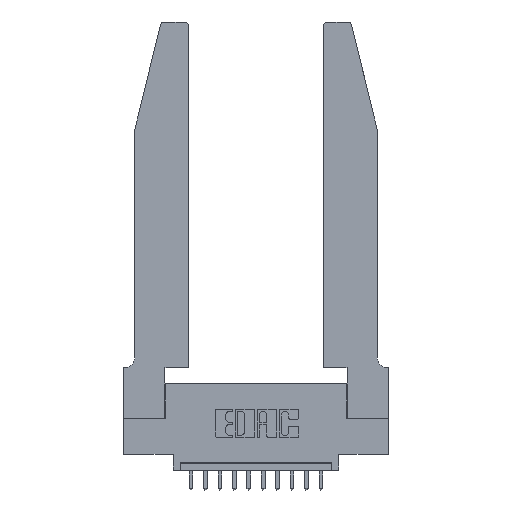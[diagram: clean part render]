
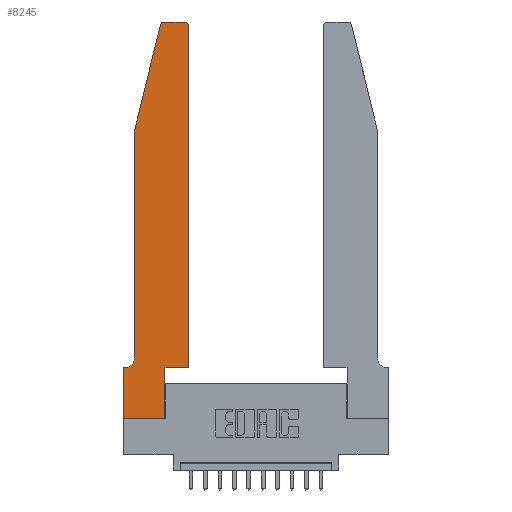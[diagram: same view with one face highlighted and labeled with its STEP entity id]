
A CAD part, top view. The second image highlights one B-rep face of the part: STEP entity #8245.
In plain terms, the highlighted planar face has unit normal (0, 0, 1).
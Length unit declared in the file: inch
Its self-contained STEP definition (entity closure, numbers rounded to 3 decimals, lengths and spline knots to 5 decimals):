
#214 = ORIENTED_EDGE ( 'NONE', *, *, #12427, .T. ) ;
#364 = CARTESIAN_POINT ( 'NONE',  ( 0.0755, 2., 0.37 ) ) ;
#446 = DIRECTION ( 'NONE',  ( -1., 0., 0. ) ) ;
#519 = EDGE_CURVE ( 'NONE', #14532, #1285, #1143, .T. ) ;
#826 = VERTEX_POINT ( 'NONE', #7293 ) ;
#1064 = VECTOR ( 'NONE', #11147, 39.37008 ) ;
#1143 = LINE ( 'NONE', #16599, #11051 ) ;
#1285 = VERTEX_POINT ( 'NONE', #364 ) ;
#1430 = VERTEX_POINT ( 'NONE', #10833 ) ;
#1676 = ORIENTED_EDGE ( 'NONE', *, *, #519, .T. ) ;
#1747 = DIRECTION ( 'NONE',  ( 1., 0., 0. ) ) ;
#1871 = DIRECTION ( 'NONE',  ( 0., 0., -1. ) ) ;
#1930 = VERTEX_POINT ( 'NONE', #14676 ) ;
#2020 = EDGE_CURVE ( 'NONE', #9613, #1430, #5554, .T. ) ;
#2262 = EDGE_CURVE ( 'NONE', #9826, #11814, #2734, .T. ) ;
#2315 = VECTOR ( 'NONE', #14000, 39.37008 ) ;
#2559 = DIRECTION ( 'NONE',  ( -0.239, -0.971, 0. ) ) ;
#2623 = CARTESIAN_POINT ( 'NONE',  ( 0.4505, 0.35, 0.37 ) ) ;
#2734 = LINE ( 'NONE', #5154, #2315 ) ;
#2771 = EDGE_CURVE ( 'NONE', #14630, #3129, #10166, .T. ) ;
#3014 = EDGE_CURVE ( 'NONE', #826, #9613, #12371, .T. ) ;
#3129 = VERTEX_POINT ( 'NONE', #7586 ) ;
#3206 = ORIENTED_EDGE ( 'NONE', *, *, #6426, .T. ) ;
#3350 = CARTESIAN_POINT ( 'NONE',  ( 0., 0., 0.37 ) ) ;
#3402 = LINE ( 'NONE', #9365, #4191 ) ;
#3431 = CARTESIAN_POINT ( 'NONE',  ( 0.25487, 2.72718, 0.37 ) ) ;
#3450 = EDGE_LOOP ( 'NONE', ( #13868, #10071, #1676, #14899, #9707, #16537, #13257, #11878, #3206, #13038, #214, #4531 ) ) ;
#3834 = VECTOR ( 'NONE', #12925, 39.37008 ) ;
#3857 = CARTESIAN_POINT ( 'NONE',  ( 0., 0.35, 0.37 ) ) ;
#3971 = CARTESIAN_POINT ( 'NONE',  ( 0.4205, 2.72, 0.37 ) ) ;
#4080 = DIRECTION ( 'NONE',  ( 0., 0., 1. ) ) ;
#4191 = VECTOR ( 'NONE', #446, 39.37008 ) ;
#4404 = EDGE_CURVE ( 'NONE', #1285, #1930, #16577, .T. ) ;
#4475 = DIRECTION ( 'NONE',  ( -1., 0., 0. ) ) ;
#4479 = CARTESIAN_POINT ( 'NONE',  ( 0., 0., 0.37 ) ) ;
#4531 = ORIENTED_EDGE ( 'NONE', *, *, #2771, .T. ) ;
#4622 = DIRECTION ( 'NONE',  ( 0., 1., 0. ) ) ;
#4669 = LINE ( 'NONE', #2623, #3834 ) ;
#5014 = DIRECTION ( 'NONE',  ( 0., 0., 1. ) ) ;
#5154 = CARTESIAN_POINT ( 'NONE',  ( 0.4505, 0.35, 0.37 ) ) ;
#5554 = LINE ( 'NONE', #3350, #15008 ) ;
#5591 = CARTESIAN_POINT ( 'NONE',  ( 0.4505, 0.35, 0.37 ) ) ;
#5852 = DIRECTION ( 'NONE',  ( 1., 0., 0. ) ) ;
#6157 = CARTESIAN_POINT ( 'NONE',  ( 0.2865, 0.35, 0.37 ) ) ;
#6426 = EDGE_CURVE ( 'NONE', #1430, #9826, #13929, .T. ) ;
#6497 = AXIS2_PLACEMENT_3D ( 'NONE', #14771, #1871, #4475 ) ;
#7072 = EDGE_CURVE ( 'NONE', #3129, #7613, #3402, .T. ) ;
#7178 = CARTESIAN_POINT ( 'NONE',  ( 0.2865, 0.35, 0.37 ) ) ;
#7293 = CARTESIAN_POINT ( 'NONE',  ( 0., 0.35, 0.37 ) ) ;
#7442 = DIRECTION ( 'NONE',  ( -1., 0., 0. ) ) ;
#7586 = CARTESIAN_POINT ( 'NONE',  ( 0.4205, 2.75, 0.37 ) ) ;
#7613 = VERTEX_POINT ( 'NONE', #16133 ) ;
#8162 = CIRCLE ( 'NONE', #6497, 0.07 ) ;
#8190 = CARTESIAN_POINT ( 'NONE',  ( 0.284, 2.72, 0.37 ) ) ;
#8245 = ADVANCED_FACE ( 'NONE', ( #15655 ), #9014, .T. ) ;
#8492 = VECTOR ( 'NONE', #12927, 39.37008 ) ;
#9014 = PLANE ( 'NONE',  #12389 ) ;
#9365 = CARTESIAN_POINT ( 'NONE',  ( 0.2605, 2.75, 0.37 ) ) ;
#9613 = VERTEX_POINT ( 'NONE', #14556 ) ;
#9707 = ORIENTED_EDGE ( 'NONE', *, *, #15686, .T. ) ;
#9826 = VERTEX_POINT ( 'NONE', #6157 ) ;
#9971 = CARTESIAN_POINT ( 'NONE',  ( 0.0755, 0.35, 0.37 ) ) ;
#10071 = ORIENTED_EDGE ( 'NONE', *, *, #15635, .T. ) ;
#10166 = CIRCLE ( 'NONE', #13939, 0.03 ) ;
#10833 = CARTESIAN_POINT ( 'NONE',  ( 0.2865, 0., 0.37 ) ) ;
#11051 = VECTOR ( 'NONE', #2559, 39.37008 ) ;
#11102 = VECTOR ( 'NONE', #4622, 39.37008 ) ;
#11147 = DIRECTION ( 'NONE',  ( 0., -1., 0. ) ) ;
#11606 = CIRCLE ( 'NONE', #14357, 0.03 ) ;
#11757 = CARTESIAN_POINT ( 'NONE',  ( 0.0755, 2., 0.37 ) ) ;
#11814 = VERTEX_POINT ( 'NONE', #5591 ) ;
#11878 = ORIENTED_EDGE ( 'NONE', *, *, #2020, .T. ) ;
#12342 = CARTESIAN_POINT ( 'NONE',  ( 0.0055, 0.35, 0.37 ) ) ;
#12371 = LINE ( 'NONE', #4479, #1064 ) ;
#12389 = AXIS2_PLACEMENT_3D ( 'NONE', #3857, #5014, #16685 ) ;
#12427 = EDGE_CURVE ( 'NONE', #11814, #14630, #4669, .T. ) ;
#12925 = DIRECTION ( 'NONE',  ( 0., 1., 0. ) ) ;
#12927 = DIRECTION ( 'NONE',  ( 0., -1., 0. ) ) ;
#13038 = ORIENTED_EDGE ( 'NONE', *, *, #2262, .T. ) ;
#13257 = ORIENTED_EDGE ( 'NONE', *, *, #3014, .T. ) ;
#13438 = DIRECTION ( 'NONE',  ( 0., 0., 1. ) ) ;
#13712 = CARTESIAN_POINT ( 'NONE',  ( 0.4505, 2.72, 0.37 ) ) ;
#13868 = ORIENTED_EDGE ( 'NONE', *, *, #7072, .T. ) ;
#13929 = LINE ( 'NONE', #7178, #11102 ) ;
#13939 = AXIS2_PLACEMENT_3D ( 'NONE', #3971, #4080, #14350 ) ;
#14000 = DIRECTION ( 'NONE',  ( 1., 0., 0. ) ) ;
#14048 = LINE ( 'NONE', #9971, #15449 ) ;
#14350 = DIRECTION ( 'NONE',  ( 1., 0., 0. ) ) ;
#14357 = AXIS2_PLACEMENT_3D ( 'NONE', #8190, #13438, #1747 ) ;
#14532 = VERTEX_POINT ( 'NONE', #3431 ) ;
#14556 = CARTESIAN_POINT ( 'NONE',  ( 0., 0., 0.37 ) ) ;
#14630 = VERTEX_POINT ( 'NONE', #13712 ) ;
#14676 = CARTESIAN_POINT ( 'NONE',  ( 0.0755, 0.42, 0.37 ) ) ;
#14771 = CARTESIAN_POINT ( 'NONE',  ( 0.0055, 0.42, 0.37 ) ) ;
#14792 = EDGE_CURVE ( 'NONE', #16671, #826, #14048, .T. ) ;
#14899 = ORIENTED_EDGE ( 'NONE', *, *, #4404, .T. ) ;
#15008 = VECTOR ( 'NONE', #5852, 39.37008 ) ;
#15449 = VECTOR ( 'NONE', #7442, 39.37008 ) ;
#15635 = EDGE_CURVE ( 'NONE', #7613, #14532, #11606, .T. ) ;
#15655 = FACE_OUTER_BOUND ( 'NONE', #3450, .T. ) ;
#15686 = EDGE_CURVE ( 'NONE', #1930, #16671, #8162, .T. ) ;
#16133 = CARTESIAN_POINT ( 'NONE',  ( 0.284, 2.75, 0.37 ) ) ;
#16537 = ORIENTED_EDGE ( 'NONE', *, *, #14792, .T. ) ;
#16577 = LINE ( 'NONE', #11757, #8492 ) ;
#16599 = CARTESIAN_POINT ( 'NONE',  ( 0.0755, 2., 0.37 ) ) ;
#16671 = VERTEX_POINT ( 'NONE', #12342 ) ;
#16685 = DIRECTION ( 'NONE',  ( 1., 0., 0. ) ) ;
